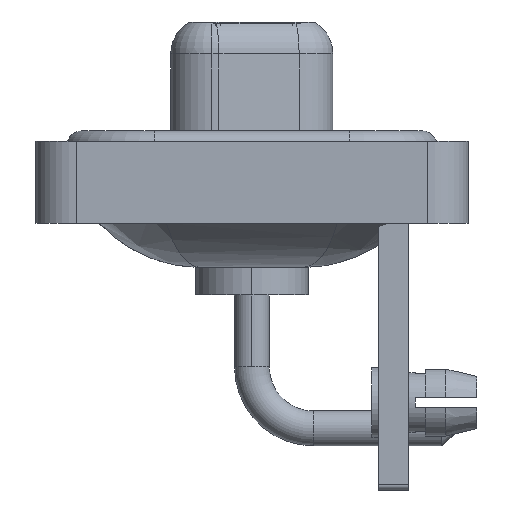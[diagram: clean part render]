
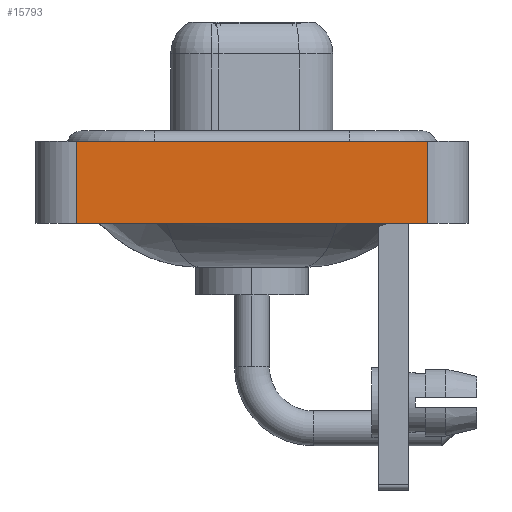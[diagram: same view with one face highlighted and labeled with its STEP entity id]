
A CAD part, left-side view. The second image highlights one B-rep face of the part: STEP entity #15793.
In plain terms, the highlighted planar face has unit normal (-1, 0, 0).
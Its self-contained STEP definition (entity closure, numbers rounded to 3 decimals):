
#386 = CARTESIAN_POINT ( 'NONE',  ( -7.25, -8.55, 0.4 ) ) ;
#934 = VERTEX_POINT ( 'NONE', #3035 ) ;
#1356 = VERTEX_POINT ( 'NONE', #14754 ) ;
#2056 = CARTESIAN_POINT ( 'NONE',  ( -7.25, 8.55, 0.4 ) ) ;
#2894 = DIRECTION ( 'NONE',  ( 0., -1., 0. ) ) ;
#3035 = CARTESIAN_POINT ( 'NONE',  ( -7.25, -8.55, 0.4 ) ) ;
#3812 = ORIENTED_EDGE ( 'NONE', *, *, #10234, .T. ) ;
#5442 = CARTESIAN_POINT ( 'NONE',  ( -7.25, -8.55, -3.6 ) ) ;
#6381 = VECTOR ( 'NONE', #2894, 1000. ) ;
#6621 = CARTESIAN_POINT ( 'NONE',  ( -7.25, -8.55, -3.6 ) ) ;
#6718 = DIRECTION ( 'NONE',  ( -1., 0., 0. ) ) ;
#7553 = AXIS2_PLACEMENT_3D ( 'NONE', #6621, #6718, #12692 ) ;
#7859 = LINE ( 'NONE', #7952, #12802 ) ;
#7952 = CARTESIAN_POINT ( 'NONE',  ( -7.25, 8.55, -3.6 ) ) ;
#8187 = DIRECTION ( 'NONE',  ( 0., 0., 1. ) ) ;
#8205 = FACE_OUTER_BOUND ( 'NONE', #18416, .T. ) ;
#9092 = VECTOR ( 'NONE', #15092, 1000. ) ;
#9244 = CARTESIAN_POINT ( 'NONE',  ( -7.25, 8.55, -3.6 ) ) ;
#10006 = EDGE_CURVE ( 'NONE', #1356, #934, #12769, .T. ) ;
#10234 = EDGE_CURVE ( 'NONE', #16111, #1356, #17752, .T. ) ;
#10332 = CARTESIAN_POINT ( 'NONE',  ( -7.25, -8.55, -3.6 ) ) ;
#10851 = ORIENTED_EDGE ( 'NONE', *, *, #10006, .T. ) ;
#10933 = VERTEX_POINT ( 'NONE', #2056 ) ;
#11079 = ORIENTED_EDGE ( 'NONE', *, *, #12201, .F. ) ;
#12201 = EDGE_CURVE ( 'NONE', #16111, #10933, #7859, .T. ) ;
#12444 = DIRECTION ( 'NONE',  ( 0., 0., 1. ) ) ;
#12692 = DIRECTION ( 'NONE',  ( 0., 0., 1. ) ) ;
#12769 = LINE ( 'NONE', #5442, #14216 ) ;
#12802 = VECTOR ( 'NONE', #12444, 1000. ) ;
#13810 = LINE ( 'NONE', #386, #9092 ) ;
#14216 = VECTOR ( 'NONE', #8187, 1000. ) ;
#14754 = CARTESIAN_POINT ( 'NONE',  ( -7.25, -8.55, -3.6 ) ) ;
#15092 = DIRECTION ( 'NONE',  ( 0., -1., 0. ) ) ;
#15279 = EDGE_CURVE ( 'NONE', #10933, #934, #13810, .T. ) ;
#15793 = ADVANCED_FACE ( 'NONE', ( #8205 ), #18471, .T. ) ;
#16111 = VERTEX_POINT ( 'NONE', #9244 ) ;
#17430 = ORIENTED_EDGE ( 'NONE', *, *, #15279, .F. ) ;
#17752 = LINE ( 'NONE', #10332, #6381 ) ;
#18416 = EDGE_LOOP ( 'NONE', ( #10851, #17430, #11079, #3812 ) ) ;
#18471 = PLANE ( 'NONE',  #7553 ) ;
